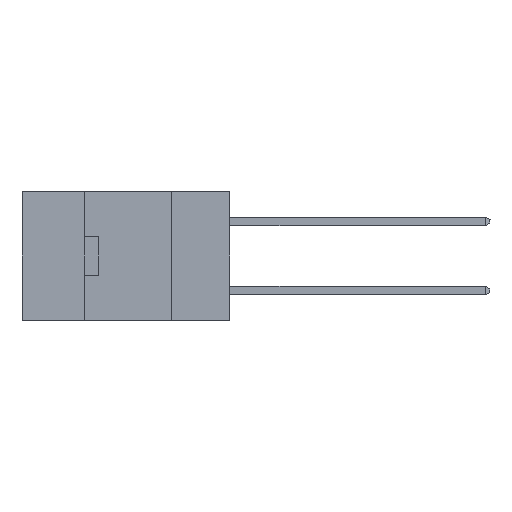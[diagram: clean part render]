
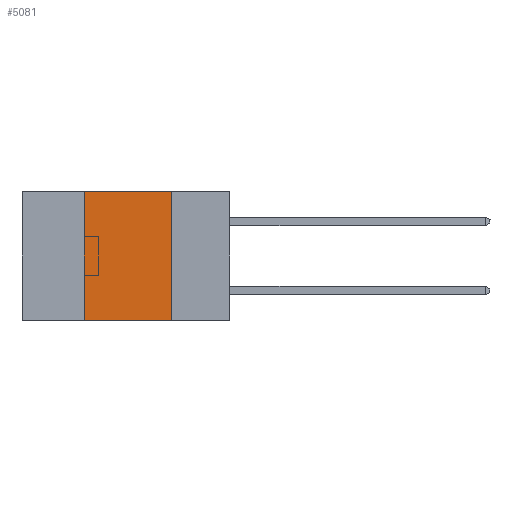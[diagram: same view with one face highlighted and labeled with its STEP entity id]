
A CAD part, left-side view. The second image highlights one B-rep face of the part: STEP entity #5081.
In plain terms, the highlighted planar face has unit normal (-1, 0, 0).
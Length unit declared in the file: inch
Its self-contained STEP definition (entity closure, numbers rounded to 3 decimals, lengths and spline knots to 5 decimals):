
#1411 = VECTOR ( 'NONE', #20803, 39.37008 ) ;
#1980 = DIRECTION ( 'NONE',  ( 0., -1., 0. ) ) ;
#3490 = VECTOR ( 'NONE', #18061, 39.37008 ) ;
#4832 = CARTESIAN_POINT ( 'NONE',  ( 0., 0.6, 0. ) ) ;
#4918 = VERTEX_POINT ( 'NONE', #22236 ) ;
#5081 = ADVANCED_FACE ( 'NONE', ( #8371 ), #27418, .F. ) ;
#6473 = CARTESIAN_POINT ( 'NONE',  ( 0., 0.17, -0.37 ) ) ;
#7218 = DIRECTION ( 'NONE',  ( 0., -1., 0. ) ) ;
#7373 = ORIENTED_EDGE ( 'NONE', *, *, #23821, .T. ) ;
#7518 = ORIENTED_EDGE ( 'NONE', *, *, #11327, .F. ) ;
#8238 = CARTESIAN_POINT ( 'NONE',  ( 0., 0.6, 0. ) ) ;
#8371 = FACE_OUTER_BOUND ( 'NONE', #19795, .T. ) ;
#9459 = VECTOR ( 'NONE', #7218, 39.37008 ) ;
#10103 = CARTESIAN_POINT ( 'NONE',  ( 0., 0.6, -0.37 ) ) ;
#10638 = LINE ( 'NONE', #6473, #3490 ) ;
#11224 = AXIS2_PLACEMENT_3D ( 'NONE', #8238, #16879, #17302 ) ;
#11327 = EDGE_CURVE ( 'NONE', #14853, #21853, #15302, .T. ) ;
#11670 = EDGE_CURVE ( 'NONE', #21853, #21608, #10638, .T. ) ;
#11902 = ORIENTED_EDGE ( 'NONE', *, *, #18649, .F. ) ;
#14853 = VERTEX_POINT ( 'NONE', #20881 ) ;
#15124 = CARTESIAN_POINT ( 'NONE',  ( 0., 0.17, 0. ) ) ;
#15302 = LINE ( 'NONE', #4832, #9459 ) ;
#15875 = VECTOR ( 'NONE', #1980, 39.37008 ) ;
#16826 = CARTESIAN_POINT ( 'NONE',  ( 0., 0.17, -0.37 ) ) ;
#16879 = DIRECTION ( 'NONE',  ( 1., 0., 0. ) ) ;
#17302 = DIRECTION ( 'NONE',  ( 0., 0., -1. ) ) ;
#18061 = DIRECTION ( 'NONE',  ( 0., 0., -1. ) ) ;
#18073 = ORIENTED_EDGE ( 'NONE', *, *, #11670, .F. ) ;
#18570 = LINE ( 'NONE', #26973, #1411 ) ;
#18649 = EDGE_CURVE ( 'NONE', #4918, #14853, #18570, .T. ) ;
#19795 = EDGE_LOOP ( 'NONE', ( #18073, #7518, #11902, #7373 ) ) ;
#20803 = DIRECTION ( 'NONE',  ( 0., 0., 1. ) ) ;
#20881 = CARTESIAN_POINT ( 'NONE',  ( 0., 0.42, 0. ) ) ;
#21608 = VERTEX_POINT ( 'NONE', #16826 ) ;
#21853 = VERTEX_POINT ( 'NONE', #15124 ) ;
#22236 = CARTESIAN_POINT ( 'NONE',  ( 0., 0.42, -0.37 ) ) ;
#23821 = EDGE_CURVE ( 'NONE', #4918, #21608, #27320, .T. ) ;
#26973 = CARTESIAN_POINT ( 'NONE',  ( 0., 0.42, -0.37 ) ) ;
#27320 = LINE ( 'NONE', #10103, #15875 ) ;
#27418 = PLANE ( 'NONE',  #11224 ) ;
